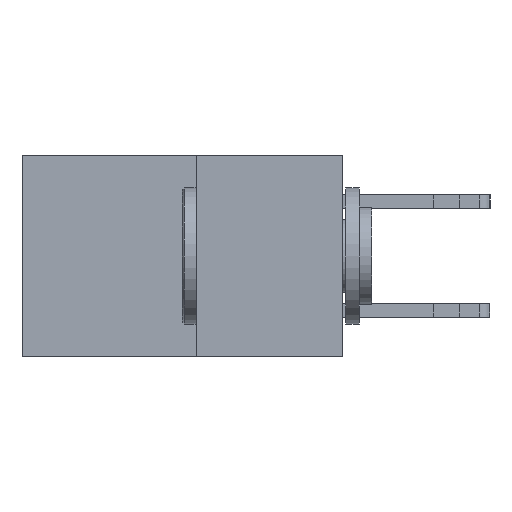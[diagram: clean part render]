
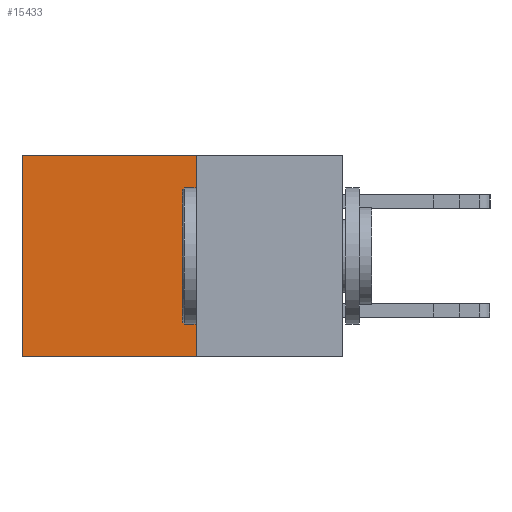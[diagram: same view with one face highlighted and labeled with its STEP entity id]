
A CAD part, left-side view. The second image highlights one B-rep face of the part: STEP entity #15433.
In plain terms, the highlighted planar face has unit normal (-1, 0, 0).
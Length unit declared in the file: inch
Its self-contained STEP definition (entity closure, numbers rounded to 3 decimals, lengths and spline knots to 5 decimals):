
#2129 = LINE ( 'NONE', #7768, #19986 ) ;
#2428 = DIRECTION ( 'NONE',  ( 0., 0., -1. ) ) ;
#3330 = VECTOR ( 'NONE', #11788, 39.37008 ) ;
#4613 = LINE ( 'NONE', #19083, #14449 ) ;
#5380 = CARTESIAN_POINT ( 'NONE',  ( 0.277, 0.27, -0.37 ) ) ;
#5986 = EDGE_CURVE ( 'NONE', #7388, #13044, #15798, .T. ) ;
#6242 = EDGE_CURVE ( 'NONE', #26485, #13044, #2129, .T. ) ;
#7308 = ORIENTED_EDGE ( 'NONE', *, *, #24337, .T. ) ;
#7388 = VERTEX_POINT ( 'NONE', #18219 ) ;
#7634 = DIRECTION ( 'NONE',  ( 0., 0., -1. ) ) ;
#7768 = CARTESIAN_POINT ( 'NONE',  ( 0.277, 0.27, -0.37 ) ) ;
#9848 = VECTOR ( 'NONE', #2428, 39.37008 ) ;
#10024 = EDGE_CURVE ( 'NONE', #18595, #26485, #27190, .T. ) ;
#11453 = ORIENTED_EDGE ( 'NONE', *, *, #10024, .F. ) ;
#11788 = DIRECTION ( 'NONE',  ( 0., 0., -1. ) ) ;
#13044 = VERTEX_POINT ( 'NONE', #15058 ) ;
#13610 = CARTESIAN_POINT ( 'NONE',  ( 0.277, 0.59, -0.37 ) ) ;
#14449 = VECTOR ( 'NONE', #23588, 39.37008 ) ;
#15058 = CARTESIAN_POINT ( 'NONE',  ( 0.277, 0.59, -0.37 ) ) ;
#15433 = ADVANCED_FACE ( 'NONE', ( #17140 ), #16570, .F. ) ;
#15798 = LINE ( 'NONE', #13610, #9848 ) ;
#16444 = ORIENTED_EDGE ( 'NONE', *, *, #6242, .F. ) ;
#16570 = PLANE ( 'NONE',  #28873 ) ;
#17140 = FACE_OUTER_BOUND ( 'NONE', #25642, .T. ) ;
#18219 = CARTESIAN_POINT ( 'NONE',  ( 0.277, 0.59, 0. ) ) ;
#18595 = VERTEX_POINT ( 'NONE', #22751 ) ;
#19083 = CARTESIAN_POINT ( 'NONE',  ( 0.277, 0.27, 0. ) ) ;
#19986 = VECTOR ( 'NONE', #23463, 39.37008 ) ;
#20808 = ORIENTED_EDGE ( 'NONE', *, *, #5986, .T. ) ;
#21057 = DIRECTION ( 'NONE',  ( 1., 0., 0. ) ) ;
#21512 = CARTESIAN_POINT ( 'NONE',  ( 0.277, 0.27, -0.37 ) ) ;
#22751 = CARTESIAN_POINT ( 'NONE',  ( 0.277, 0.27, 0. ) ) ;
#23463 = DIRECTION ( 'NONE',  ( 0., 1., 0. ) ) ;
#23588 = DIRECTION ( 'NONE',  ( 0., 1., 0. ) ) ;
#24337 = EDGE_CURVE ( 'NONE', #18595, #7388, #4613, .T. ) ;
#25642 = EDGE_LOOP ( 'NONE', ( #20808, #16444, #11453, #7308 ) ) ;
#26485 = VERTEX_POINT ( 'NONE', #21512 ) ;
#27190 = LINE ( 'NONE', #27478, #3330 ) ;
#27478 = CARTESIAN_POINT ( 'NONE',  ( 0.277, 0.27, -0.37 ) ) ;
#28873 = AXIS2_PLACEMENT_3D ( 'NONE', #5380, #21057, #7634 ) ;
